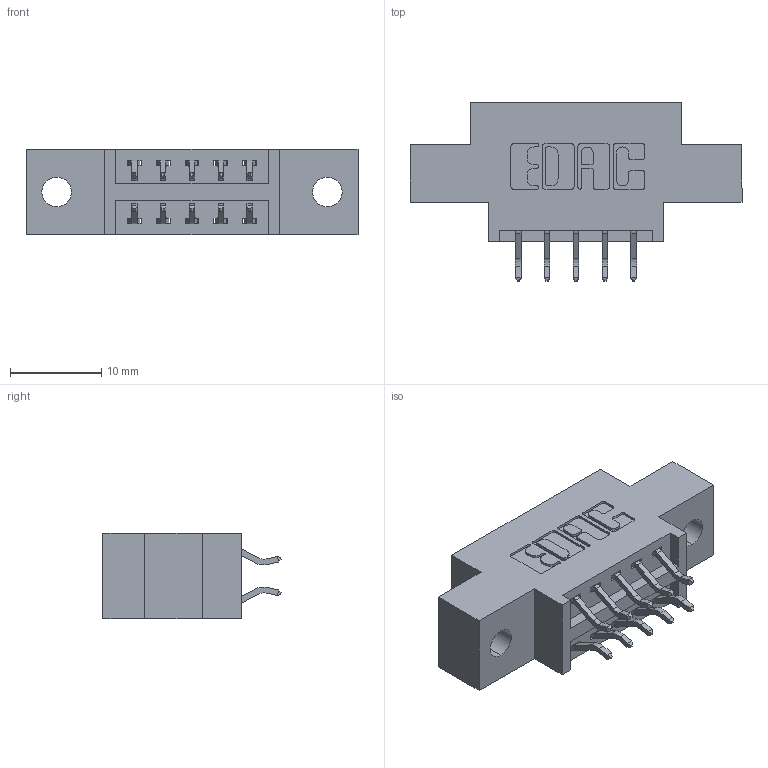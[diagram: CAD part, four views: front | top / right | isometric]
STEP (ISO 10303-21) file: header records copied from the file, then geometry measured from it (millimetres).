
FILE_DESCRIPTION (( 'STEP AP203' ), '1' );
FILE_NAME ('396-010-556-802.STEP', '2019-11-01T16:50:12', ( '' ), ( '' ), 'SwSTEP 2.0', 'SolidWorks 2016', '' );
FILE_SCHEMA (( 'CONFIG_CONTROL_DESIGN' ));
Length unit declared in the file: inch
Products named in the file (3): 346 Part_0.170 Offset - 0.128 Dia; 345-292-001_556 Tail; 396-010-556-802
Assembly tree (11 placements, depth 2):
  396-010-556-802
    346 Part_0.170 Offset - 0.128 Dia
    345-292-001_556 Tail  x10
Bounding box: 36.45 x 19.57 x 9.4 mm (x, y, z)
Volume: 3075.2 mm3; surface area: 3546.6 mm2
Topology: 11 solids, 11 shells, 706 faces, 2071 edges, 1366 vertices
Faces by surface type: plane 470, cylinder 236
Entity records: 8599 total; most frequent: CARTESIAN_POINT 1484, ORIENTED_EDGE 1406, DIRECTION 1347, EDGE_CURVE 703, VECTOR 543, LINE 543, VERTEX_POINT 466, AXIS2_PLACEMENT_3D 402
